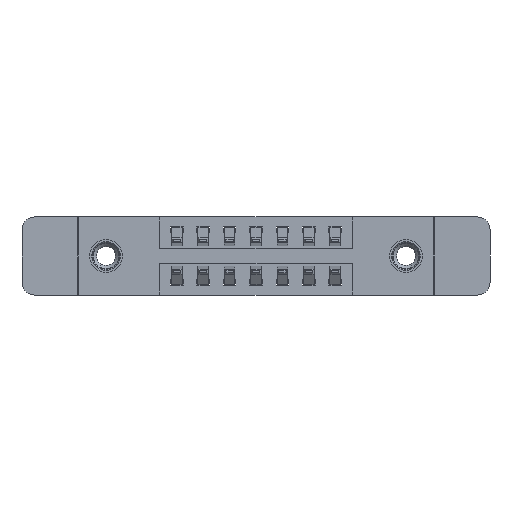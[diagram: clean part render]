
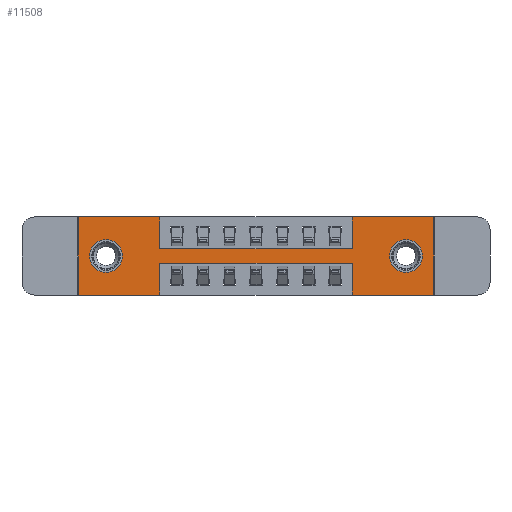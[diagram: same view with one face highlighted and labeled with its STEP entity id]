
A CAD part, front view. The second image highlights one B-rep face of the part: STEP entity #11508.
In plain terms, the highlighted planar face has unit normal (0, -1, 0).
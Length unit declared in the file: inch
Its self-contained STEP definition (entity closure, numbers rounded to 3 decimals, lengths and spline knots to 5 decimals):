
#146 = DIRECTION ( 'NONE',  ( 0., 0., 1. ) ) ;
#204 = DIRECTION ( 'NONE',  ( 0., 0., 1. ) ) ;
#373 = EDGE_CURVE ( 'NONE', #7301, #6955, #2626, .T. ) ;
#527 = CARTESIAN_POINT ( 'NONE',  ( 0., 0., 0. ) ) ;
#678 = VECTOR ( 'NONE', #11110, 39.37008 ) ;
#782 = VERTEX_POINT ( 'NONE', #4230 ) ;
#1016 = DIRECTION ( 'NONE',  ( 1., 0., 0. ) ) ;
#1091 = LINE ( 'NONE', #1658, #4595 ) ;
#1146 = CARTESIAN_POINT ( 'NONE',  ( 0.1325, 0., -0.263 ) ) ;
#1308 = LINE ( 'NONE', #7749, #3929 ) ;
#1468 = EDGE_CURVE ( 'NONE', #12513, #3752, #6637, .T. ) ;
#1622 = AXIS2_PLACEMENT_3D ( 'NONE', #9953, #9759, #12337 ) ;
#1635 = ORIENTED_EDGE ( 'NONE', *, *, #1468, .T. ) ;
#1658 = CARTESIAN_POINT ( 'NONE',  ( 0., 0., -0.37 ) ) ;
#1720 = CIRCLE ( 'NONE', #13586, 0.078 ) ;
#1749 = FACE_BOUND ( 'NONE', #2294, .T. ) ;
#2019 = CARTESIAN_POINT ( 'NONE',  ( 1.2975, 0., -0.37 ) ) ;
#2154 = VECTOR ( 'NONE', #146, 39.37008 ) ;
#2294 = EDGE_LOOP ( 'NONE', ( #11210, #1635 ) ) ;
#2560 = EDGE_CURVE ( 'NONE', #3849, #13509, #9605, .T. ) ;
#2574 = VERTEX_POINT ( 'NONE', #3536 ) ;
#2626 = CIRCLE ( 'NONE', #5555, 0.078 ) ;
#2804 = CARTESIAN_POINT ( 'NONE',  ( 0., 0., 0. ) ) ;
#3069 = DIRECTION ( 'NONE',  ( 0., 0., -1. ) ) ;
#3300 = VECTOR ( 'NONE', #8138, 39.37008 ) ;
#3399 = CARTESIAN_POINT ( 'NONE',  ( 1.2975, 0., 0. ) ) ;
#3536 = CARTESIAN_POINT ( 'NONE',  ( 1.685, 0., 0. ) ) ;
#3752 = VERTEX_POINT ( 'NONE', #9589 ) ;
#3763 = CARTESIAN_POINT ( 'NONE',  ( 0., 0., -0.37 ) ) ;
#3836 = VECTOR ( 'NONE', #9714, 39.37008 ) ;
#3849 = VERTEX_POINT ( 'NONE', #9784 ) ;
#3929 = VECTOR ( 'NONE', #1016, 39.37008 ) ;
#3958 = CARTESIAN_POINT ( 'NONE',  ( 1.2975, 0., 0. ) ) ;
#4230 = CARTESIAN_POINT ( 'NONE',  ( 1.2975, 0., -0.15 ) ) ;
#4281 = VECTOR ( 'NONE', #3069, 39.37008 ) ;
#4440 = LINE ( 'NONE', #3958, #12570 ) ;
#4449 = DIRECTION ( 'NONE',  ( 0., 1., 0. ) ) ;
#4550 = LINE ( 'NONE', #13266, #678 ) ;
#4595 = VECTOR ( 'NONE', #8414, 39.37008 ) ;
#4759 = FACE_BOUND ( 'NONE', #5297, .T. ) ;
#4974 = DIRECTION ( 'NONE',  ( 0., 1., 0. ) ) ;
#4975 = EDGE_CURVE ( 'NONE', #12001, #782, #1308, .T. ) ;
#5145 = EDGE_CURVE ( 'NONE', #7158, #12689, #10818, .T. ) ;
#5187 = CARTESIAN_POINT ( 'NONE',  ( 1.5525, 0., -0.263 ) ) ;
#5212 = ORIENTED_EDGE ( 'NONE', *, *, #13168, .F. ) ;
#5297 = EDGE_LOOP ( 'NONE', ( #5365, #11179 ) ) ;
#5298 = VERTEX_POINT ( 'NONE', #10856 ) ;
#5365 = ORIENTED_EDGE ( 'NONE', *, *, #13593, .T. ) ;
#5399 = VECTOR ( 'NONE', #9614, 39.37008 ) ;
#5455 = ORIENTED_EDGE ( 'NONE', *, *, #13673, .F. ) ;
#5499 = ORIENTED_EDGE ( 'NONE', *, *, #2560, .F. ) ;
#5555 = AXIS2_PLACEMENT_3D ( 'NONE', #8524, #4974, #13056 ) ;
#5634 = ORIENTED_EDGE ( 'NONE', *, *, #8047, .F. ) ;
#5645 = ORIENTED_EDGE ( 'NONE', *, *, #5145, .F. ) ;
#5808 = EDGE_CURVE ( 'NONE', #782, #8442, #4440, .T. ) ;
#5832 = LINE ( 'NONE', #7909, #13441 ) ;
#6009 = EDGE_CURVE ( 'NONE', #6388, #12001, #5832, .T. ) ;
#6034 = AXIS2_PLACEMENT_3D ( 'NONE', #3763, #12782, #13917 ) ;
#6053 = CARTESIAN_POINT ( 'NONE',  ( 1.2975, 0., -0.37 ) ) ;
#6114 = ORIENTED_EDGE ( 'NONE', *, *, #4975, .F. ) ;
#6388 = VERTEX_POINT ( 'NONE', #12200 ) ;
#6453 = CARTESIAN_POINT ( 'NONE',  ( 0.3875, 0., -0.22 ) ) ;
#6637 = CIRCLE ( 'NONE', #1622, 0.078 ) ;
#6662 = DIRECTION ( 'NONE',  ( 0., 0., -1. ) ) ;
#6687 = EDGE_CURVE ( 'NONE', #10572, #7158, #1091, .T. ) ;
#6717 = CARTESIAN_POINT ( 'NONE',  ( 0., 0., 0. ) ) ;
#6866 = ORIENTED_EDGE ( 'NONE', *, *, #6687, .F. ) ;
#6955 = VERTEX_POINT ( 'NONE', #11038 ) ;
#6978 = CARTESIAN_POINT ( 'NONE',  ( 0., 0., -0.37 ) ) ;
#6986 = ORIENTED_EDGE ( 'NONE', *, *, #5808, .F. ) ;
#7123 = PLANE ( 'NONE',  #6034 ) ;
#7126 = DIRECTION ( 'NONE',  ( 0., 1., 0. ) ) ;
#7158 = VERTEX_POINT ( 'NONE', #11004 ) ;
#7301 = VERTEX_POINT ( 'NONE', #5187 ) ;
#7413 = ORIENTED_EDGE ( 'NONE', *, *, #13967, .F. ) ;
#7448 = EDGE_CURVE ( 'NONE', #3752, #12513, #9507, .T. ) ;
#7749 = CARTESIAN_POINT ( 'NONE',  ( 0.3875, 0., -0.15 ) ) ;
#7754 = FACE_OUTER_BOUND ( 'NONE', #9132, .T. ) ;
#7909 = CARTESIAN_POINT ( 'NONE',  ( 0.3875, 0., 0. ) ) ;
#7921 = VECTOR ( 'NONE', #13634, 39.37008 ) ;
#8047 = EDGE_CURVE ( 'NONE', #13490, #3849, #11268, .T. ) ;
#8138 = DIRECTION ( 'NONE',  ( 1., 0., 0. ) ) ;
#8186 = EDGE_CURVE ( 'NONE', #13509, #10572, #4550, .T. ) ;
#8414 = DIRECTION ( 'NONE',  ( -1., 0., 0. ) ) ;
#8442 = VERTEX_POINT ( 'NONE', #3399 ) ;
#8524 = CARTESIAN_POINT ( 'NONE',  ( 1.5525, 0., -0.185 ) ) ;
#8736 = VECTOR ( 'NONE', #12464, 39.37008 ) ;
#9132 = EDGE_LOOP ( 'NONE', ( #12420, #5499, #5634, #5212, #13681, #7413, #6986, #6114, #11201, #5455, #5645, #6866 ) ) ;
#9223 = CARTESIAN_POINT ( 'NONE',  ( 0.3875, 0., -0.15 ) ) ;
#9507 = CIRCLE ( 'NONE', #13984, 0.078 ) ;
#9509 = CARTESIAN_POINT ( 'NONE',  ( 0.3875, 0., -0.37 ) ) ;
#9589 = CARTESIAN_POINT ( 'NONE',  ( 0.1325, 0., -0.107 ) ) ;
#9605 = LINE ( 'NONE', #12519, #8736 ) ;
#9614 = DIRECTION ( 'NONE',  ( 1., 0., 0. ) ) ;
#9714 = DIRECTION ( 'NONE',  ( 0., 0., 1. ) ) ;
#9759 = DIRECTION ( 'NONE',  ( 0., 1., 0. ) ) ;
#9760 = EDGE_CURVE ( 'NONE', #2574, #5298, #12231, .T. ) ;
#9784 = CARTESIAN_POINT ( 'NONE',  ( 1.2975, 0., -0.22 ) ) ;
#9953 = CARTESIAN_POINT ( 'NONE',  ( 0.1325, 0., -0.185 ) ) ;
#10355 = CARTESIAN_POINT ( 'NONE',  ( 1.5525, 0., -0.185 ) ) ;
#10572 = VERTEX_POINT ( 'NONE', #9509 ) ;
#10818 = LINE ( 'NONE', #6717, #2154 ) ;
#10856 = CARTESIAN_POINT ( 'NONE',  ( 1.685, 0., -0.37 ) ) ;
#11004 = CARTESIAN_POINT ( 'NONE',  ( 0., 0., -0.37 ) ) ;
#11038 = CARTESIAN_POINT ( 'NONE',  ( 1.5525, 0., -0.107 ) ) ;
#11110 = DIRECTION ( 'NONE',  ( 0., 0., -1. ) ) ;
#11179 = ORIENTED_EDGE ( 'NONE', *, *, #373, .T. ) ;
#11201 = ORIENTED_EDGE ( 'NONE', *, *, #6009, .F. ) ;
#11210 = ORIENTED_EDGE ( 'NONE', *, *, #7448, .T. ) ;
#11246 = LINE ( 'NONE', #11507, #3300 ) ;
#11268 = LINE ( 'NONE', #6053, #3836 ) ;
#11430 = LINE ( 'NONE', #527, #5399 ) ;
#11507 = CARTESIAN_POINT ( 'NONE',  ( 0., 0., 0. ) ) ;
#11508 = ADVANCED_FACE ( 'NONE', ( #4759, #1749, #7754 ), #7123, .T. ) ;
#11618 = CARTESIAN_POINT ( 'NONE',  ( 0.1325, 0., -0.185 ) ) ;
#11996 = CARTESIAN_POINT ( 'NONE',  ( 1.685, 0., 0. ) ) ;
#12001 = VERTEX_POINT ( 'NONE', #9223 ) ;
#12200 = CARTESIAN_POINT ( 'NONE',  ( 0.3875, 0., 0. ) ) ;
#12231 = LINE ( 'NONE', #11996, #4281 ) ;
#12337 = DIRECTION ( 'NONE',  ( 0., 0., 1. ) ) ;
#12420 = ORIENTED_EDGE ( 'NONE', *, *, #8186, .F. ) ;
#12464 = DIRECTION ( 'NONE',  ( -1., 0., 0. ) ) ;
#12513 = VERTEX_POINT ( 'NONE', #1146 ) ;
#12519 = CARTESIAN_POINT ( 'NONE',  ( 0.3875, 0., -0.22 ) ) ;
#12570 = VECTOR ( 'NONE', #13324, 39.37008 ) ;
#12689 = VERTEX_POINT ( 'NONE', #2804 ) ;
#12782 = DIRECTION ( 'NONE',  ( 0., -1., 0. ) ) ;
#13056 = DIRECTION ( 'NONE',  ( 0., 0., -1. ) ) ;
#13168 = EDGE_CURVE ( 'NONE', #5298, #13490, #13901, .T. ) ;
#13266 = CARTESIAN_POINT ( 'NONE',  ( 0.3875, 0., -0.37 ) ) ;
#13324 = DIRECTION ( 'NONE',  ( 0., 0., 1. ) ) ;
#13441 = VECTOR ( 'NONE', #13578, 39.37008 ) ;
#13490 = VERTEX_POINT ( 'NONE', #2019 ) ;
#13509 = VERTEX_POINT ( 'NONE', #6453 ) ;
#13578 = DIRECTION ( 'NONE',  ( 0., 0., -1. ) ) ;
#13586 = AXIS2_PLACEMENT_3D ( 'NONE', #10355, #4449, #6662 ) ;
#13593 = EDGE_CURVE ( 'NONE', #6955, #7301, #1720, .T. ) ;
#13634 = DIRECTION ( 'NONE',  ( -1., 0., 0. ) ) ;
#13673 = EDGE_CURVE ( 'NONE', #12689, #6388, #11246, .T. ) ;
#13681 = ORIENTED_EDGE ( 'NONE', *, *, #9760, .F. ) ;
#13901 = LINE ( 'NONE', #6978, #7921 ) ;
#13917 = DIRECTION ( 'NONE',  ( 0., 0., -1. ) ) ;
#13967 = EDGE_CURVE ( 'NONE', #8442, #2574, #11430, .T. ) ;
#13984 = AXIS2_PLACEMENT_3D ( 'NONE', #11618, #7126, #204 ) ;
